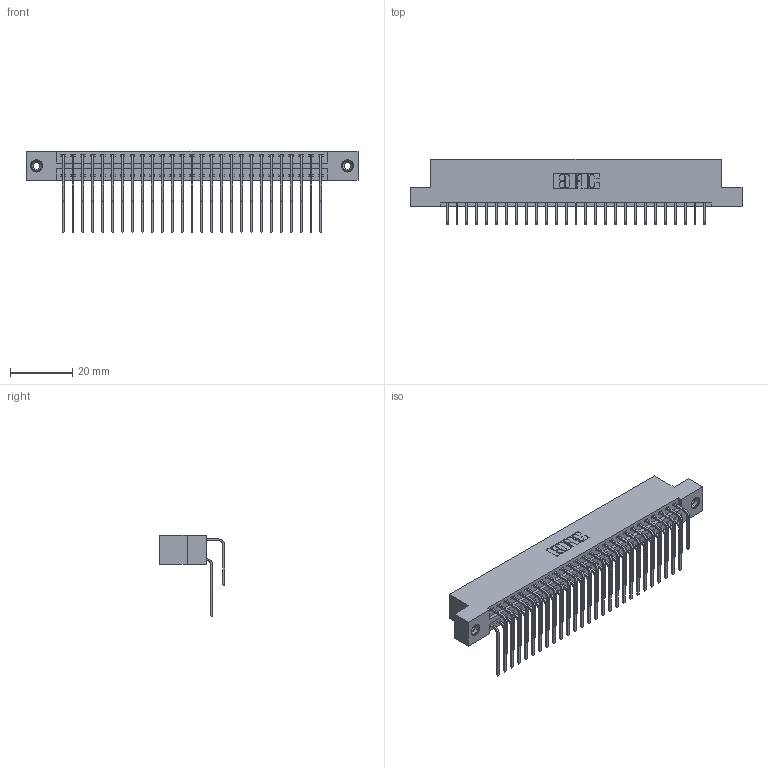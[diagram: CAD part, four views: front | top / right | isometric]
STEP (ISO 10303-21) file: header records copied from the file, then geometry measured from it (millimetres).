
FILE_DESCRIPTION (( 'STEP AP203' ), '1' );
FILE_NAME ('396-054-559-208.STEP', '2018-09-08T08:46:17', ( '' ), ( '' ), 'SwSTEP 2.0', 'SolidWorks 2016', '' );
FILE_SCHEMA (( 'CONFIG_CONTROL_DESIGN' ));
Length unit declared in the file: inch
Products named in the file (5): 346 Part_Flush Mounting Lugs - 0.156 Dia-TI; 345-292-001_558 559 Tail - 1; 345-292-001_559 Tail - 2; 345-250-001_345-250-003-102; 396-054-559-208
Assembly tree (57 placements, depth 2):
  396-054-559-208
    346 Part_Flush Mounting Lugs - 0.156 Dia-TI
    345-292-001_558 559 Tail - 1  x27
    345-292-001_559 Tail - 2  x27
    345-250-001_345-250-003-102  x2
Bounding box: 106.3 x 20.89 x 26.16 mm (x, y, z)
Volume: 10554 mm3; surface area: 15785.8 mm2
Topology: 57 solids, 57 shells, 3098 faces, 9159 edges, 6026 vertices
Faces by surface type: plane 2106, cylinder 976, cone 12, torus 4
Entity records: 22610 total; most frequent: CARTESIAN_POINT 3782, ORIENTED_EDGE 3658, DIRECTION 3383, EDGE_CURVE 1829, VECTOR 1529, LINE 1529, VERTEX_POINT 1212, AXIS2_PLACEMENT_3D 927
